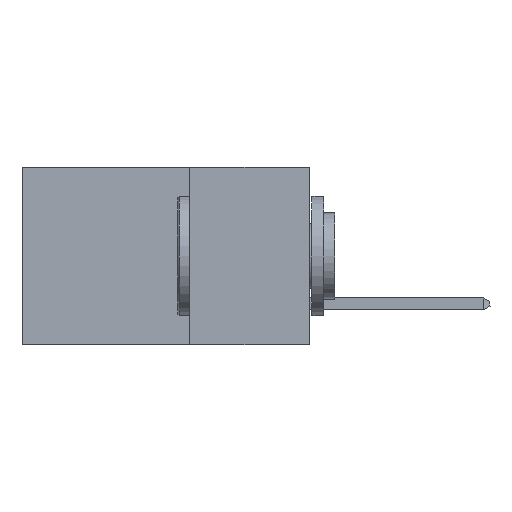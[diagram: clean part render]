
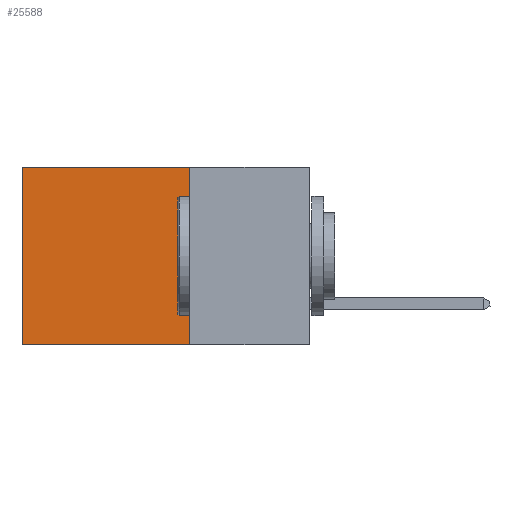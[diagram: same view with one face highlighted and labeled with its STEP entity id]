
A CAD part, left-side view. The second image highlights one B-rep face of the part: STEP entity #25588.
In plain terms, the highlighted planar face has unit normal (-1, 0, 0).
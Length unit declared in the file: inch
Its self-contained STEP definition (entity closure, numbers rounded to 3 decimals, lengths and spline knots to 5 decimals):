
#449 = EDGE_LOOP ( 'NONE', ( #18295, #10463, #12548, #35730 ) ) ;
#958 = DIRECTION ( 'NONE',  ( 0., 1., 0. ) ) ;
#2502 = DIRECTION ( 'NONE',  ( 0., 0., -1. ) ) ;
#3069 = VERTEX_POINT ( 'NONE', #24349 ) ;
#3202 = CARTESIAN_POINT ( 'NONE',  ( 0.2875, 0.25, 0. ) ) ;
#3966 = DIRECTION ( 'NONE',  ( 0., 1., 0. ) ) ;
#5620 = LINE ( 'NONE', #28500, #19770 ) ;
#6079 = DIRECTION ( 'NONE',  ( 1., 0., 0. ) ) ;
#8469 = VECTOR ( 'NONE', #2502, 39.37008 ) ;
#9030 = VERTEX_POINT ( 'NONE', #9602 ) ;
#9602 = CARTESIAN_POINT ( 'NONE',  ( 0.2875, 0.6, -0.37 ) ) ;
#10463 = ORIENTED_EDGE ( 'NONE', *, *, #25120, .F. ) ;
#11275 = LINE ( 'NONE', #29319, #17882 ) ;
#12548 = ORIENTED_EDGE ( 'NONE', *, *, #22646, .F. ) ;
#13002 = AXIS2_PLACEMENT_3D ( 'NONE', #3202, #6079, #25833 ) ;
#13414 = CARTESIAN_POINT ( 'NONE',  ( 0.2875, 0.25, -0.37 ) ) ;
#13654 = EDGE_CURVE ( 'NONE', #3069, #36604, #14750, .T. ) ;
#13823 = CARTESIAN_POINT ( 'NONE',  ( 0.2875, 0.6, 0. ) ) ;
#14633 = EDGE_CURVE ( 'NONE', #36604, #9030, #25230, .T. ) ;
#14750 = LINE ( 'NONE', #34817, #28859 ) ;
#17882 = VECTOR ( 'NONE', #3966, 39.37008 ) ;
#18295 = ORIENTED_EDGE ( 'NONE', *, *, #14633, .T. ) ;
#19770 = VECTOR ( 'NONE', #31313, 39.37008 ) ;
#20021 = CARTESIAN_POINT ( 'NONE',  ( 0.2875, 0.6, 0. ) ) ;
#21790 = VERTEX_POINT ( 'NONE', #13414 ) ;
#22646 = EDGE_CURVE ( 'NONE', #3069, #21790, #5620, .T. ) ;
#24349 = CARTESIAN_POINT ( 'NONE',  ( 0.2875, 0.25, 0. ) ) ;
#25120 = EDGE_CURVE ( 'NONE', #21790, #9030, #11275, .T. ) ;
#25230 = LINE ( 'NONE', #13823, #8469 ) ;
#25588 = ADVANCED_FACE ( 'NONE', ( #26567 ), #31383, .F. ) ;
#25833 = DIRECTION ( 'NONE',  ( 0., 0., -1. ) ) ;
#26567 = FACE_OUTER_BOUND ( 'NONE', #449, .T. ) ;
#28500 = CARTESIAN_POINT ( 'NONE',  ( 0.2875, 0.25, 0. ) ) ;
#28859 = VECTOR ( 'NONE', #958, 39.37008 ) ;
#29319 = CARTESIAN_POINT ( 'NONE',  ( 0.2875, 0.25, -0.37 ) ) ;
#31313 = DIRECTION ( 'NONE',  ( 0., 0., -1. ) ) ;
#31383 = PLANE ( 'NONE',  #13002 ) ;
#34817 = CARTESIAN_POINT ( 'NONE',  ( 0.2875, 0.25, 0. ) ) ;
#35730 = ORIENTED_EDGE ( 'NONE', *, *, #13654, .T. ) ;
#36604 = VERTEX_POINT ( 'NONE', #20021 ) ;
